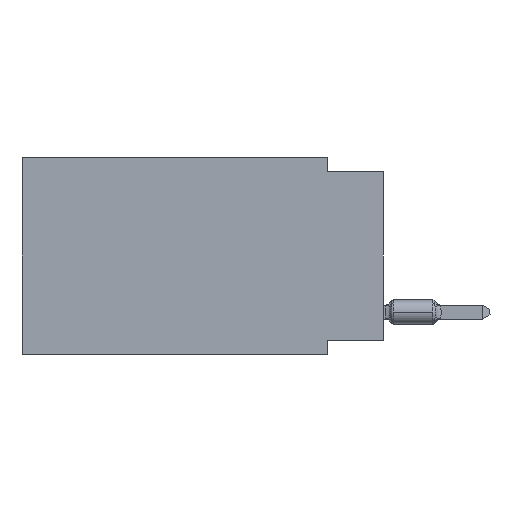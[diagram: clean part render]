
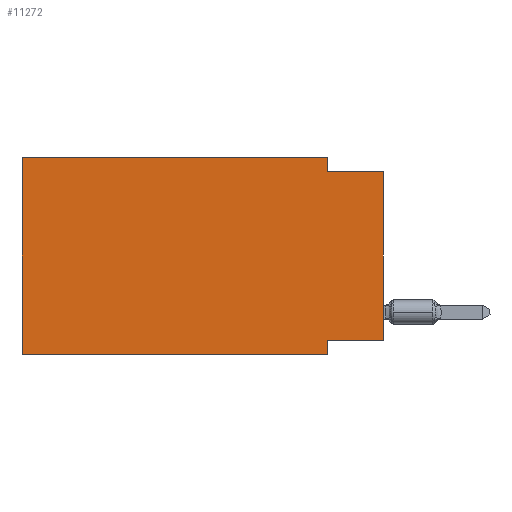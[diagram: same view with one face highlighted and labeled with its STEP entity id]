
A CAD part, left-side view. The second image highlights one B-rep face of the part: STEP entity #11272.
In plain terms, the highlighted planar face has unit normal (-1, 0, 0).
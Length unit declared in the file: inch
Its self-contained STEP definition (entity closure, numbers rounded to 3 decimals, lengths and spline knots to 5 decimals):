
#3 = PLANE ( 'NONE',  #3402 ) ;
#129 = DIRECTION ( 'NONE',  ( 0., 1., 0. ) ) ;
#295 = CARTESIAN_POINT ( 'NONE',  ( 0., 0.1, 0. ) ) ;
#311 = CARTESIAN_POINT ( 'NONE',  ( 0., 0.645, 0. ) ) ;
#704 = CARTESIAN_POINT ( 'NONE',  ( 0., 0.645, 0. ) ) ;
#806 = ORIENTED_EDGE ( 'NONE', *, *, #3998, .T. ) ;
#946 = DIRECTION ( 'NONE',  ( 0., 0., 1. ) ) ;
#953 = DIRECTION ( 'NONE',  ( 0., 0., -1. ) ) ;
#2039 = LINE ( 'NONE', #6192, #10249 ) ;
#2765 = ORIENTED_EDGE ( 'NONE', *, *, #3574, .T. ) ;
#2984 = ORIENTED_EDGE ( 'NONE', *, *, #12730, .F. ) ;
#3011 = LINE ( 'NONE', #7168, #9915 ) ;
#3402 = AXIS2_PLACEMENT_3D ( 'NONE', #4155, #9473, #9408 ) ;
#3410 = CARTESIAN_POINT ( 'NONE',  ( 0., 0.1, 0. ) ) ;
#3574 = EDGE_CURVE ( 'NONE', #9124, #8607, #3011, .T. ) ;
#3971 = EDGE_CURVE ( 'NONE', #6369, #10139, #6259, .T. ) ;
#3998 = EDGE_CURVE ( 'NONE', #11098, #10139, #2039, .T. ) ;
#4084 = CARTESIAN_POINT ( 'NONE',  ( 0., 0.1, -0.35 ) ) ;
#4144 = VECTOR ( 'NONE', #946, 39.37008 ) ;
#4155 = CARTESIAN_POINT ( 'NONE',  ( 0., 0.645, 0. ) ) ;
#4346 = CARTESIAN_POINT ( 'NONE',  ( 0., 0., -0.325 ) ) ;
#4556 = EDGE_CURVE ( 'NONE', #11098, #5063, #12391, .T. ) ;
#4832 = ORIENTED_EDGE ( 'NONE', *, *, #8733, .F. ) ;
#4865 = ORIENTED_EDGE ( 'NONE', *, *, #11270, .F. ) ;
#5063 = VERTEX_POINT ( 'NONE', #311 ) ;
#5240 = CARTESIAN_POINT ( 'NONE',  ( 0., 0.645, 0. ) ) ;
#5307 = FACE_OUTER_BOUND ( 'NONE', #5353, .T. ) ;
#5334 = LINE ( 'NONE', #9501, #13292 ) ;
#5353 = EDGE_LOOP ( 'NONE', ( #2765, #8457, #4832, #4865, #9015, #806, #12341, #2984 ) ) ;
#5613 = VERTEX_POINT ( 'NONE', #295 ) ;
#6192 = CARTESIAN_POINT ( 'NONE',  ( 0., 0.645, -0.35 ) ) ;
#6258 = LINE ( 'NONE', #10631, #13117 ) ;
#6259 = LINE ( 'NONE', #4084, #12848 ) ;
#6369 = VERTEX_POINT ( 'NONE', #8441 ) ;
#7168 = CARTESIAN_POINT ( 'NONE',  ( 0., 0., 0. ) ) ;
#7221 = DIRECTION ( 'NONE',  ( 0., -1., 0. ) ) ;
#7777 = LINE ( 'NONE', #3410, #9377 ) ;
#8261 = DIRECTION ( 'NONE',  ( 0., 0., 1. ) ) ;
#8441 = CARTESIAN_POINT ( 'NONE',  ( 0., 0.1, -0.325 ) ) ;
#8457 = ORIENTED_EDGE ( 'NONE', *, *, #9390, .F. ) ;
#8607 = VERTEX_POINT ( 'NONE', #9487 ) ;
#8733 = EDGE_CURVE ( 'NONE', #5613, #13001, #7777, .T. ) ;
#9015 = ORIENTED_EDGE ( 'NONE', *, *, #4556, .F. ) ;
#9124 = VERTEX_POINT ( 'NONE', #4346 ) ;
#9377 = VECTOR ( 'NONE', #11940, 39.37008 ) ;
#9390 = EDGE_CURVE ( 'NONE', #13001, #8607, #5334, .T. ) ;
#9408 = DIRECTION ( 'NONE',  ( 0., 0., -1. ) ) ;
#9473 = DIRECTION ( 'NONE',  ( 1., 0., 0. ) ) ;
#9487 = CARTESIAN_POINT ( 'NONE',  ( 0., 0., -0.025 ) ) ;
#9499 = VECTOR ( 'NONE', #7221, 39.37008 ) ;
#9501 = CARTESIAN_POINT ( 'NONE',  ( 0., 0., -0.025 ) ) ;
#9915 = VECTOR ( 'NONE', #8261, 39.37008 ) ;
#10014 = CARTESIAN_POINT ( 'NONE',  ( 0., 0.1, -0.025 ) ) ;
#10139 = VERTEX_POINT ( 'NONE', #11584 ) ;
#10249 = VECTOR ( 'NONE', #10365, 39.37008 ) ;
#10365 = DIRECTION ( 'NONE',  ( 0., -1., 0. ) ) ;
#10631 = CARTESIAN_POINT ( 'NONE',  ( 0., 0., -0.325 ) ) ;
#11098 = VERTEX_POINT ( 'NONE', #13356 ) ;
#11270 = EDGE_CURVE ( 'NONE', #5063, #5613, #12466, .T. ) ;
#11272 = ADVANCED_FACE ( 'NONE', ( #5307 ), #3, .F. ) ;
#11584 = CARTESIAN_POINT ( 'NONE',  ( 0., 0.1, -0.35 ) ) ;
#11686 = DIRECTION ( 'NONE',  ( 0., -1., 0. ) ) ;
#11940 = DIRECTION ( 'NONE',  ( 0., 0., -1. ) ) ;
#12341 = ORIENTED_EDGE ( 'NONE', *, *, #3971, .F. ) ;
#12391 = LINE ( 'NONE', #704, #4144 ) ;
#12466 = LINE ( 'NONE', #5240, #9499 ) ;
#12730 = EDGE_CURVE ( 'NONE', #9124, #6369, #6258, .T. ) ;
#12848 = VECTOR ( 'NONE', #953, 39.37008 ) ;
#13001 = VERTEX_POINT ( 'NONE', #10014 ) ;
#13117 = VECTOR ( 'NONE', #129, 39.37008 ) ;
#13292 = VECTOR ( 'NONE', #11686, 39.37008 ) ;
#13356 = CARTESIAN_POINT ( 'NONE',  ( 0., 0.645, -0.35 ) ) ;
